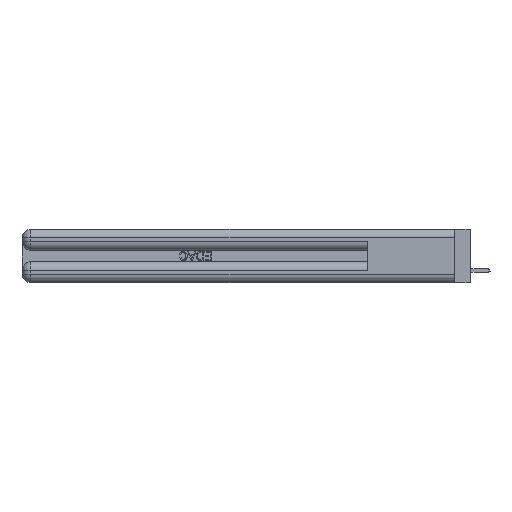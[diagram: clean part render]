
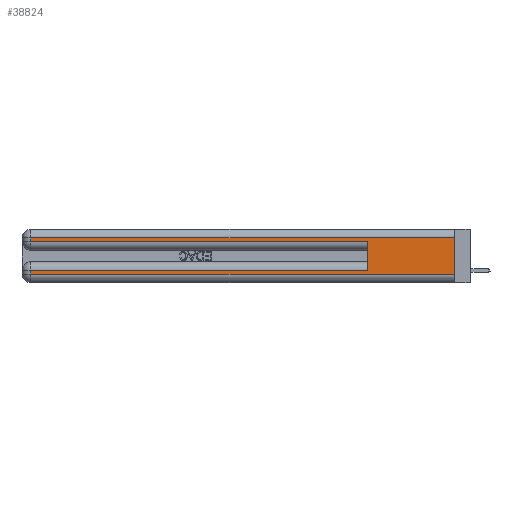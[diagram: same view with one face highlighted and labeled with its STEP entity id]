
A CAD part, left-side view. The second image highlights one B-rep face of the part: STEP entity #38824.
In plain terms, the highlighted planar face has unit normal (-1, 0, 0).
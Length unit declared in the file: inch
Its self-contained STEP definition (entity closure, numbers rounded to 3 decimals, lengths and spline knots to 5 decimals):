
#226 = VERTEX_POINT ( 'NONE', #35232 ) ;
#464 = VECTOR ( 'NONE', #41548, 39.37008 ) ;
#705 = VERTEX_POINT ( 'NONE', #15491 ) ;
#979 = VERTEX_POINT ( 'NONE', #28225 ) ;
#1056 = VERTEX_POINT ( 'NONE', #32198 ) ;
#2297 = FACE_OUTER_BOUND ( 'NONE', #19643, .T. ) ;
#2793 = LINE ( 'NONE', #34033, #44999 ) ;
#3183 = LINE ( 'NONE', #42054, #3791 ) ;
#3785 = PLANE ( 'NONE',  #23488 ) ;
#3791 = VECTOR ( 'NONE', #50798, 39.37008 ) ;
#3793 = LINE ( 'NONE', #20469, #47322 ) ;
#4914 = LINE ( 'NONE', #44803, #464 ) ;
#7036 = CARTESIAN_POINT ( 'NONE',  ( 0., 0., 0.06 ) ) ;
#8279 = LINE ( 'NONE', #25598, #26089 ) ;
#10874 = DIRECTION ( 'NONE',  ( 0., 0., 1. ) ) ;
#11210 = VECTOR ( 'NONE', #41285, 39.37008 ) ;
#11218 = CARTESIAN_POINT ( 'NONE',  ( 0., 0.6, 0.145 ) ) ;
#12901 = ORIENTED_EDGE ( 'NONE', *, *, #36332, .T. ) ;
#13442 = VERTEX_POINT ( 'NONE', #7036 ) ;
#14378 = LINE ( 'NONE', #37152, #11210 ) ;
#15491 = CARTESIAN_POINT ( 'NONE',  ( 0., 2.94, 0.085 ) ) ;
#17528 = VERTEX_POINT ( 'NONE', #52658 ) ;
#17619 = VERTEX_POINT ( 'NONE', #22209 ) ;
#19643 = EDGE_LOOP ( 'NONE', ( #26415, #41249, #12901, #20470, #42820, #36901, #36414, #46603 ) ) ;
#19825 = VERTEX_POINT ( 'NONE', #47326 ) ;
#20469 = CARTESIAN_POINT ( 'NONE',  ( 0., 0., 0.37 ) ) ;
#20470 = ORIENTED_EDGE ( 'NONE', *, *, #36339, .T. ) ;
#22209 = CARTESIAN_POINT ( 'NONE',  ( 0., 2.94, 0.06 ) ) ;
#23488 = AXIS2_PLACEMENT_3D ( 'NONE', #24463, #41327, #41821 ) ;
#23976 = EDGE_CURVE ( 'NONE', #979, #226, #37158, .T. ) ;
#24234 = DIRECTION ( 'NONE',  ( 0., 0., -1. ) ) ;
#24463 = CARTESIAN_POINT ( 'NONE',  ( 0., 0., 0.37 ) ) ;
#25030 = EDGE_CURVE ( 'NONE', #979, #705, #4914, .T. ) ;
#25598 = CARTESIAN_POINT ( 'NONE',  ( 0., 0., 0.31 ) ) ;
#26089 = VECTOR ( 'NONE', #50541, 39.37008 ) ;
#26415 = ORIENTED_EDGE ( 'NONE', *, *, #43432, .F. ) ;
#28071 = LINE ( 'NONE', #51168, #47320 ) ;
#28225 = CARTESIAN_POINT ( 'NONE',  ( 0., 0.6, 0.085 ) ) ;
#30759 = DIRECTION ( 'NONE',  ( 0., -1., 0. ) ) ;
#32198 = CARTESIAN_POINT ( 'NONE',  ( 0., 0., 0.31 ) ) ;
#34033 = CARTESIAN_POINT ( 'NONE',  ( 0., 2.94, 0.37 ) ) ;
#35232 = CARTESIAN_POINT ( 'NONE',  ( 0., 0.6, 0.285 ) ) ;
#36332 = EDGE_CURVE ( 'NONE', #19825, #17528, #3183, .T. ) ;
#36339 = EDGE_CURVE ( 'NONE', #17528, #226, #28071, .T. ) ;
#36414 = ORIENTED_EDGE ( 'NONE', *, *, #50662, .T. ) ;
#36901 = ORIENTED_EDGE ( 'NONE', *, *, #25030, .T. ) ;
#37152 = CARTESIAN_POINT ( 'NONE',  ( 0., 0., 0.06 ) ) ;
#37158 = LINE ( 'NONE', #11218, #44230 ) ;
#38824 = ADVANCED_FACE ( 'NONE', ( #2297 ), #3785, .F. ) ;
#41249 = ORIENTED_EDGE ( 'NONE', *, *, #43121, .T. ) ;
#41285 = DIRECTION ( 'NONE',  ( 0., -1., 0. ) ) ;
#41327 = DIRECTION ( 'NONE',  ( 1., 0., 0. ) ) ;
#41548 = DIRECTION ( 'NONE',  ( 0., 1., 0. ) ) ;
#41821 = DIRECTION ( 'NONE',  ( 0., 0., -1. ) ) ;
#42054 = CARTESIAN_POINT ( 'NONE',  ( 0., 2.94, 0.37 ) ) ;
#42659 = DIRECTION ( 'NONE',  ( 0., 0., -1. ) ) ;
#42820 = ORIENTED_EDGE ( 'NONE', *, *, #23976, .F. ) ;
#43121 = EDGE_CURVE ( 'NONE', #1056, #19825, #8279, .T. ) ;
#43432 = EDGE_CURVE ( 'NONE', #1056, #13442, #3793, .T. ) ;
#44230 = VECTOR ( 'NONE', #10874, 39.37008 ) ;
#44803 = CARTESIAN_POINT ( 'NONE',  ( 0., 0., 0.085 ) ) ;
#44999 = VECTOR ( 'NONE', #42659, 39.37008 ) ;
#46603 = ORIENTED_EDGE ( 'NONE', *, *, #49285, .T. ) ;
#47320 = VECTOR ( 'NONE', #30759, 39.37008 ) ;
#47322 = VECTOR ( 'NONE', #24234, 39.37008 ) ;
#47326 = CARTESIAN_POINT ( 'NONE',  ( 0., 2.94, 0.31 ) ) ;
#49285 = EDGE_CURVE ( 'NONE', #17619, #13442, #14378, .T. ) ;
#50541 = DIRECTION ( 'NONE',  ( 0., 1., 0. ) ) ;
#50662 = EDGE_CURVE ( 'NONE', #705, #17619, #2793, .T. ) ;
#50798 = DIRECTION ( 'NONE',  ( 0., 0., -1. ) ) ;
#51168 = CARTESIAN_POINT ( 'NONE',  ( 0., 0., 0.285 ) ) ;
#52658 = CARTESIAN_POINT ( 'NONE',  ( 0., 2.94, 0.285 ) ) ;
